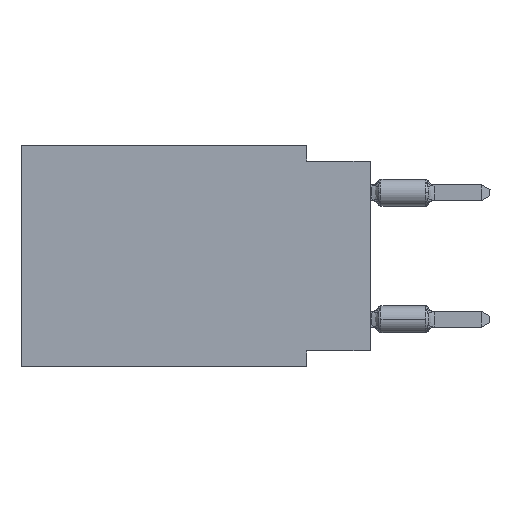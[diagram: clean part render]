
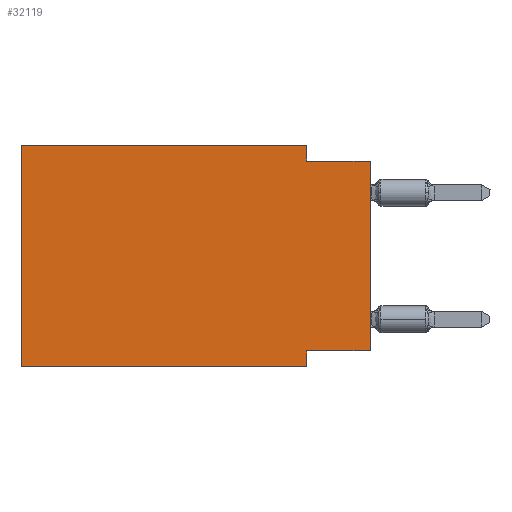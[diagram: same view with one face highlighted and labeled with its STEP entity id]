
A CAD part, left-side view. The second image highlights one B-rep face of the part: STEP entity #32119.
In plain terms, the highlighted planar face has unit normal (-1, 0, 0).
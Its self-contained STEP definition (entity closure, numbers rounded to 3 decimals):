
#420 = PLANE ( 'NONE',  #21659 ) ;
#609 = DIRECTION ( 'NONE',  ( 0., 0., -1. ) ) ;
#823 = LINE ( 'NONE', #7365, #23605 ) ;
#1416 = LINE ( 'NONE', #13892, #36791 ) ;
#2004 = VECTOR ( 'NONE', #35351, 1000. ) ;
#2139 = ORIENTED_EDGE ( 'NONE', *, *, #23116, .F. ) ;
#2926 = ORIENTED_EDGE ( 'NONE', *, *, #34382, .F. ) ;
#3271 = CARTESIAN_POINT ( 'NONE',  ( 0., 2.54, -8.89 ) ) ;
#3693 = CARTESIAN_POINT ( 'NONE',  ( 0., 13.97, 0. ) ) ;
#3702 = DIRECTION ( 'NONE',  ( 0., 0., -1. ) ) ;
#3918 = VECTOR ( 'NONE', #27057, 1000. ) ;
#4115 = CARTESIAN_POINT ( 'NONE',  ( 0., 0., -8.255 ) ) ;
#4946 = CARTESIAN_POINT ( 'NONE',  ( 0., 13.97, 0. ) ) ;
#5528 = CARTESIAN_POINT ( 'NONE',  ( 0., 13.97, 0. ) ) ;
#6515 = ORIENTED_EDGE ( 'NONE', *, *, #29397, .F. ) ;
#6662 = DIRECTION ( 'NONE',  ( 0., 0., 1. ) ) ;
#7365 = CARTESIAN_POINT ( 'NONE',  ( 0., 13.97, 0. ) ) ;
#7744 = DIRECTION ( 'NONE',  ( 0., 0., -1. ) ) ;
#8513 = ORIENTED_EDGE ( 'NONE', *, *, #10884, .T. ) ;
#8647 = CARTESIAN_POINT ( 'NONE',  ( 0., 0., -0.635 ) ) ;
#8791 = ORIENTED_EDGE ( 'NONE', *, *, #19583, .T. ) ;
#9377 = VECTOR ( 'NONE', #21105, 1000. ) ;
#9591 = ORIENTED_EDGE ( 'NONE', *, *, #12753, .F. ) ;
#10090 = VECTOR ( 'NONE', #39928, 1000. ) ;
#10884 = EDGE_CURVE ( 'NONE', #20552, #39581, #25876, .T. ) ;
#12453 = CARTESIAN_POINT ( 'NONE',  ( 0., 2.54, 0. ) ) ;
#12753 = EDGE_CURVE ( 'NONE', #19466, #30946, #1416, .T. ) ;
#13892 = CARTESIAN_POINT ( 'NONE',  ( 0., 2.54, 0. ) ) ;
#14591 = CARTESIAN_POINT ( 'NONE',  ( 0., 0., -8.255 ) ) ;
#17674 = VECTOR ( 'NONE', #3702, 1000. ) ;
#18823 = LINE ( 'NONE', #34191, #17674 ) ;
#18932 = EDGE_CURVE ( 'NONE', #36147, #19466, #32987, .T. ) ;
#19428 = DIRECTION ( 'NONE',  ( 1., 0., 0. ) ) ;
#19466 = VERTEX_POINT ( 'NONE', #12453 ) ;
#19583 = EDGE_CURVE ( 'NONE', #27576, #28182, #31688, .T. ) ;
#19884 = ORIENTED_EDGE ( 'NONE', *, *, #32127, .F. ) ;
#20552 = VERTEX_POINT ( 'NONE', #4115 ) ;
#21105 = DIRECTION ( 'NONE',  ( 0., -1., 0. ) ) ;
#21659 = AXIS2_PLACEMENT_3D ( 'NONE', #3693, #19428, #609 ) ;
#23116 = EDGE_CURVE ( 'NONE', #20552, #26223, #36276, .T. ) ;
#23605 = VECTOR ( 'NONE', #28832, 1000. ) ;
#25318 = CARTESIAN_POINT ( 'NONE',  ( 0., 13.97, -8.89 ) ) ;
#25876 = LINE ( 'NONE', #34684, #27378 ) ;
#26223 = VERTEX_POINT ( 'NONE', #26373 ) ;
#26373 = CARTESIAN_POINT ( 'NONE',  ( 0., 2.54, -8.255 ) ) ;
#27057 = DIRECTION ( 'NONE',  ( 0., 1., 0. ) ) ;
#27378 = VECTOR ( 'NONE', #6662, 1000. ) ;
#27576 = VERTEX_POINT ( 'NONE', #33811 ) ;
#28182 = VERTEX_POINT ( 'NONE', #3271 ) ;
#28832 = DIRECTION ( 'NONE',  ( 0., 0., 1. ) ) ;
#29397 = EDGE_CURVE ( 'NONE', #26223, #28182, #18823, .T. ) ;
#30946 = VERTEX_POINT ( 'NONE', #35729 ) ;
#31688 = LINE ( 'NONE', #25318, #2004 ) ;
#32119 = ADVANCED_FACE ( 'NONE', ( #36140 ), #420, .F. ) ;
#32127 = EDGE_CURVE ( 'NONE', #27576, #36147, #823, .T. ) ;
#32837 = CARTESIAN_POINT ( 'NONE',  ( 0., 0., -0.635 ) ) ;
#32987 = LINE ( 'NONE', #4946, #10090 ) ;
#33811 = CARTESIAN_POINT ( 'NONE',  ( 0., 13.97, -8.89 ) ) ;
#34191 = CARTESIAN_POINT ( 'NONE',  ( 0., 2.54, -8.89 ) ) ;
#34382 = EDGE_CURVE ( 'NONE', #30946, #39581, #36662, .T. ) ;
#34684 = CARTESIAN_POINT ( 'NONE',  ( 0., 0., 0. ) ) ;
#35351 = DIRECTION ( 'NONE',  ( 0., -1., 0. ) ) ;
#35729 = CARTESIAN_POINT ( 'NONE',  ( 0., 2.54, -0.635 ) ) ;
#35929 = EDGE_LOOP ( 'NONE', ( #8513, #2926, #9591, #38462, #19884, #8791, #6515, #2139 ) ) ;
#36140 = FACE_OUTER_BOUND ( 'NONE', #35929, .T. ) ;
#36147 = VERTEX_POINT ( 'NONE', #5528 ) ;
#36276 = LINE ( 'NONE', #14591, #3918 ) ;
#36662 = LINE ( 'NONE', #8647, #9377 ) ;
#36791 = VECTOR ( 'NONE', #7744, 1000. ) ;
#38462 = ORIENTED_EDGE ( 'NONE', *, *, #18932, .F. ) ;
#39581 = VERTEX_POINT ( 'NONE', #32837 ) ;
#39928 = DIRECTION ( 'NONE',  ( 0., -1., 0. ) ) ;
